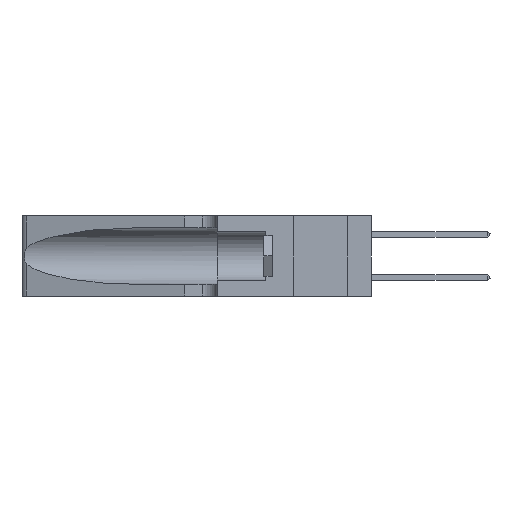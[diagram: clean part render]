
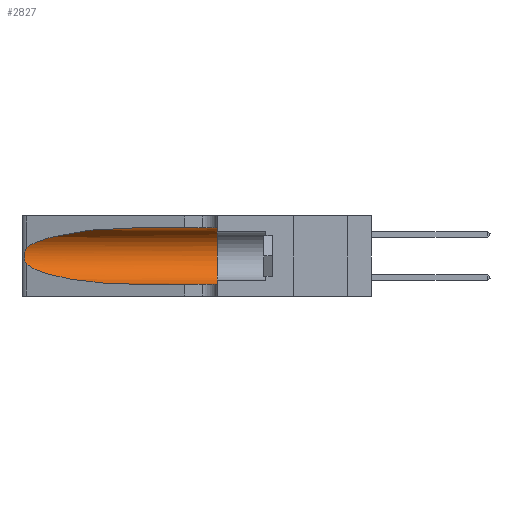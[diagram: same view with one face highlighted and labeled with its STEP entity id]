
A CAD part, left-side view. The second image highlights one B-rep face of the part: STEP entity #2827.
In plain terms, the highlighted cylindrical face has radius 3.308 mm (diameter 6.617 mm), a partial arc.
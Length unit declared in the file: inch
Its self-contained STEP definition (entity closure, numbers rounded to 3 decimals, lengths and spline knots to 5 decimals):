
#430 = VERTEX_POINT ( 'NONE', #11939 ) ;
#585 = CARTESIAN_POINT ( 'NONE',  ( 0.25787, 1.23484, 0.2124 ) ) ;
#1039 = EDGE_CURVE ( 'NONE', #12278, #7761, #24500, .T. ) ;
#1435 = CARTESIAN_POINT ( 'NONE',  ( 0.1305, 0.35, 0.185 ) ) ;
#2301 = CARTESIAN_POINT ( 'NONE',  ( 0.25487, 1.22718, 0.14631 ) ) ;
#2827 = ADVANCED_FACE ( 'NONE', ( #25547 ), #5772, .F. ) ;
#3596 =( BOUNDED_CURVE ( )  B_SPLINE_CURVE ( 3, ( #29094, #10661, #47842, #22058 ),
 .UNSPECIFIED., .F., .F. ) 
 B_SPLINE_CURVE_WITH_KNOTS ( ( 4, 4 ),
 ( 1.5708, 2.84003 ),
 .UNSPECIFIED. ) 
 CURVE ( )  GEOMETRIC_REPRESENTATION_ITEM ( )  RATIONAL_B_SPLINE_CURVE ( ( 1., 0.87, 0.87, 1. ) ) 
 REPRESENTATION_ITEM ( '' )  );
#4655 = VECTOR ( 'NONE', #7977, 39.37008 ) ;
#4678 = DIRECTION ( 'NONE',  ( 0., 1., 0. ) ) ;
#5772 = CYLINDRICAL_SURFACE ( 'NONE', #40508, 0.13025 ) ;
#5851 = CARTESIAN_POINT ( 'NONE',  ( 0.25487, 1.22718, 0.14631 ) ) ;
#6981 = VERTEX_POINT ( 'NONE', #19540 ) ;
#7444 = CARTESIAN_POINT ( 'NONE',  ( 0.25555, 1.22993, 0.14849 ) ) ;
#7671 = ORIENTED_EDGE ( 'NONE', *, *, #25457, .F. ) ;
#7758 = CARTESIAN_POINT ( 'NONE',  ( 0.25487, 1.22718, 0.14631 ) ) ;
#7761 = VERTEX_POINT ( 'NONE', #38170 ) ;
#7977 = DIRECTION ( 'NONE',  ( 0., -1., 0. ) ) ;
#9019 = ORIENTED_EDGE ( 'NONE', *, *, #22445, .T. ) ;
#9829 = ORIENTED_EDGE ( 'NONE', *, *, #34255, .T. ) ;
#10399 = VECTOR ( 'NONE', #25527, 39.37008 ) ;
#10661 = CARTESIAN_POINT ( 'NONE',  ( 0.18966, 0.96281, 0.31525 ) ) ;
#11008 = CARTESIAN_POINT ( 'NONE',  ( 0.26075, 1.23896, 0.178 ) ) ;
#11174 = CARTESIAN_POINT ( 'NONE',  ( 0.1305, 1.61858, 0.05475 ) ) ;
#11349 = CARTESIAN_POINT ( 'NONE',  ( 0.25487, 1.22718, 0.22369 ) ) ;
#11939 = CARTESIAN_POINT ( 'NONE',  ( 0.1305, 0.72297, 0.31525 ) ) ;
#12278 = VERTEX_POINT ( 'NONE', #5851 ) ;
#12913 = CARTESIAN_POINT ( 'NONE',  ( 0.1305, 0.72297, 0.05475 ) ) ;
#13543 = CARTESIAN_POINT ( 'NONE',  ( 0.2373, 1.15595, 0.08982 ) ) ;
#14561 = LINE ( 'NONE', #15306, #4655 ) ;
#14798 = CARTESIAN_POINT ( 'NONE',  ( 0.25639, 1.23184, 0.21858 ) ) ;
#14954 = CARTESIAN_POINT ( 'NONE',  ( 0.25639, 1.23186, 0.15144 ) ) ;
#15306 = CARTESIAN_POINT ( 'NONE',  ( 0.1305, 1.61858, 0.31525 ) ) ;
#15431 = CARTESIAN_POINT ( 'NONE',  ( 0.25555, 1.22994, 0.2215 ) ) ;
#15901 = DIRECTION ( 'NONE',  ( 0., 0., 1. ) ) ;
#16070 = EDGE_LOOP ( 'NONE', ( #37840, #9019, #46922, #9829, #7671, #18219 ) ) ;
#16775 = VERTEX_POINT ( 'NONE', #45633 ) ;
#16823 = LINE ( 'NONE', #11174, #10399 ) ;
#18219 = ORIENTED_EDGE ( 'NONE', *, *, #26585, .F. ) ;
#19172 = CARTESIAN_POINT ( 'NONE',  ( 0.18966, 0.96281, 0.05475 ) ) ;
#19540 = CARTESIAN_POINT ( 'NONE',  ( 0.25487, 1.22718, 0.22369 ) ) ;
#22008 = CARTESIAN_POINT ( 'NONE',  ( 0.25856, 1.23593, 0.16098 ) ) ;
#22058 = CARTESIAN_POINT ( 'NONE',  ( 0.25487, 1.22718, 0.22369 ) ) ;
#22257 = CARTESIAN_POINT ( 'NONE',  ( 0.26018, 1.23835, 0.19895 ) ) ;
#22445 = EDGE_CURVE ( 'NONE', #6981, #12278, #44822, .T. ) ;
#24500 =( BOUNDED_CURVE ( )  B_SPLINE_CURVE ( 3, ( #2301, #13543, #19172, #12913 ),
 .UNSPECIFIED., .F., .T. ) 
 B_SPLINE_CURVE_WITH_KNOTS ( ( 4, 4 ),
 ( 3.44316, 4.71239 ),
 .UNSPECIFIED. ) 
 CURVE ( )  GEOMETRIC_REPRESENTATION_ITEM ( )  RATIONAL_B_SPLINE_CURVE ( ( 1., 0.87, 0.87, 1. ) ) 
 REPRESENTATION_ITEM ( '' )  );
#25457 = EDGE_CURVE ( 'NONE', #37496, #16775, #44999, .T. ) ;
#25527 = DIRECTION ( 'NONE',  ( 0., -1., 0. ) ) ;
#25547 = FACE_OUTER_BOUND ( 'NONE', #16070, .T. ) ;
#26585 = EDGE_CURVE ( 'NONE', #430, #37496, #14561, .T. ) ;
#26645 = CARTESIAN_POINT ( 'NONE',  ( 0.26075, 1.23896, 0.19203 ) ) ;
#26743 = AXIS2_PLACEMENT_3D ( 'NONE', #1435, #4678, #15901 ) ;
#29094 = CARTESIAN_POINT ( 'NONE',  ( 0.1305, 0.72297, 0.31525 ) ) ;
#29755 = EDGE_CURVE ( 'NONE', #430, #6981, #3596, .T. ) ;
#30075 = CARTESIAN_POINT ( 'NONE',  ( 0.26017, 1.23833, 0.17102 ) ) ;
#34255 = EDGE_CURVE ( 'NONE', #7761, #16775, #16823, .T. ) ;
#34459 = CARTESIAN_POINT ( 'NONE',  ( 0.1305, 0.35, 0.31525 ) ) ;
#37496 = VERTEX_POINT ( 'NONE', #34459 ) ;
#37840 = ORIENTED_EDGE ( 'NONE', *, *, #29755, .T. ) ;
#38170 = CARTESIAN_POINT ( 'NONE',  ( 0.1305, 0.72297, 0.05475 ) ) ;
#38397 = DIRECTION ( 'NONE',  ( 0., 0., -1. ) ) ;
#38563 = DIRECTION ( 'NONE',  ( 0., -1., 0. ) ) ;
#40508 = AXIS2_PLACEMENT_3D ( 'NONE', #42337, #38563, #38397 ) ;
#41484 = CARTESIAN_POINT ( 'NONE',  ( 0.25854, 1.2359, 0.20912 ) ) ;
#42337 = CARTESIAN_POINT ( 'NONE',  ( 0.1305, 1.61858, 0.185 ) ) ;
#44770 = CARTESIAN_POINT ( 'NONE',  ( 0.25789, 1.23486, 0.15765 ) ) ;
#44822 = B_SPLINE_CURVE_WITH_KNOTS ( 'NONE', 3,
 ( #11349, #15431, #14798, #585, #41484, #22257, #26645, #11008, #30075, #22008, #44770, #14954, #7444, #7758 ),
 .UNSPECIFIED., .F., .F.,
 ( 4, 2, 2, 2, 2, 2, 4 ),
 ( 0., 0.00027, 0.00053, 0.00107, 0.0016, 0.00187, 0.00214 ),
 .UNSPECIFIED. ) ;
#44999 = CIRCLE ( 'NONE', #26743, 0.13025 ) ;
#45633 = CARTESIAN_POINT ( 'NONE',  ( 0.1305, 0.35, 0.05475 ) ) ;
#46922 = ORIENTED_EDGE ( 'NONE', *, *, #1039, .T. ) ;
#47842 = CARTESIAN_POINT ( 'NONE',  ( 0.2373, 1.15595, 0.28018 ) ) ;
